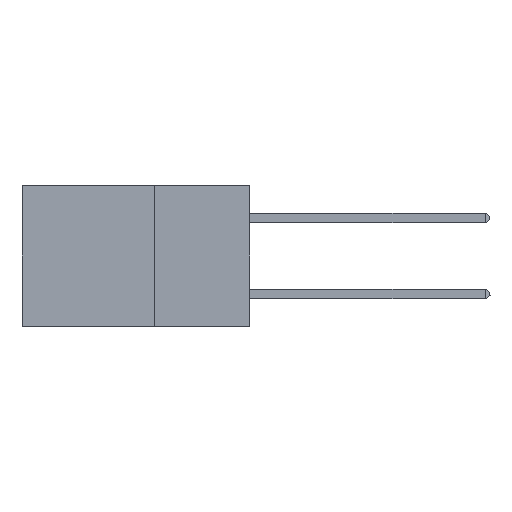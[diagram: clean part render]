
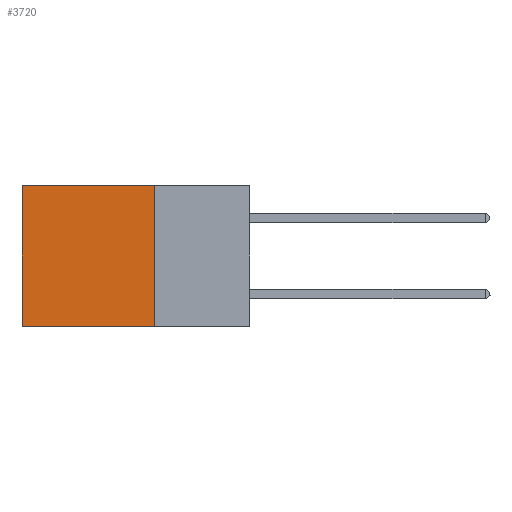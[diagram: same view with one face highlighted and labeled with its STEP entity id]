
A CAD part, left-side view. The second image highlights one B-rep face of the part: STEP entity #3720.
In plain terms, the highlighted planar face has unit normal (-1, 0, 0).
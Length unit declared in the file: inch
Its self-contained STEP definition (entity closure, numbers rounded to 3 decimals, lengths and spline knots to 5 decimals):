
#134 = AXIS2_PLACEMENT_3D ( 'NONE', #7249, #31932, #17650 ) ;
#166 = DIRECTION ( 'NONE',  ( 0., 1., 0. ) ) ;
#2289 = LINE ( 'NONE', #3078, #29446 ) ;
#2624 = DIRECTION ( 'NONE',  ( 0., 0., -1. ) ) ;
#3078 = CARTESIAN_POINT ( 'NONE',  ( 0.2875, 0.6, 0. ) ) ;
#3720 = ADVANCED_FACE ( 'NONE', ( #19783 ), #28200, .F. ) ;
#4526 = LINE ( 'NONE', #14279, #24523 ) ;
#5958 = DIRECTION ( 'NONE',  ( 0., 0., -1. ) ) ;
#6497 = CARTESIAN_POINT ( 'NONE',  ( 0.2875, 0.25, -0.37 ) ) ;
#6656 = VERTEX_POINT ( 'NONE', #38641 ) ;
#6936 = LINE ( 'NONE', #45559, #13033 ) ;
#7249 = CARTESIAN_POINT ( 'NONE',  ( 0.2875, 0.25, 0. ) ) ;
#12676 = VERTEX_POINT ( 'NONE', #6497 ) ;
#13033 = VECTOR ( 'NONE', #32696, 39.37008 ) ;
#14279 = CARTESIAN_POINT ( 'NONE',  ( 0.2875, 0.25, -0.37 ) ) ;
#15276 = CARTESIAN_POINT ( 'NONE',  ( 0.2875, 0.6, -0.37 ) ) ;
#17650 = DIRECTION ( 'NONE',  ( 0., 0., -1. ) ) ;
#19783 = FACE_OUTER_BOUND ( 'NONE', #35398, .T. ) ;
#24523 = VECTOR ( 'NONE', #166, 39.37008 ) ;
#24844 = ORIENTED_EDGE ( 'NONE', *, *, #31701, .T. ) ;
#25284 = EDGE_CURVE ( 'NONE', #12676, #30657, #4526, .T. ) ;
#25399 = LINE ( 'NONE', #26927, #41994 ) ;
#26927 = CARTESIAN_POINT ( 'NONE',  ( 0.2875, 0.25, 0. ) ) ;
#27238 = EDGE_CURVE ( 'NONE', #33437, #12676, #25399, .T. ) ;
#28200 = PLANE ( 'NONE',  #134 ) ;
#29446 = VECTOR ( 'NONE', #2624, 39.37008 ) ;
#30657 = VERTEX_POINT ( 'NONE', #15276 ) ;
#31381 = CARTESIAN_POINT ( 'NONE',  ( 0.2875, 0.25, 0. ) ) ;
#31701 = EDGE_CURVE ( 'NONE', #33437, #6656, #6936, .T. ) ;
#31932 = DIRECTION ( 'NONE',  ( 1., 0., 0. ) ) ;
#32696 = DIRECTION ( 'NONE',  ( 0., 1., 0. ) ) ;
#33437 = VERTEX_POINT ( 'NONE', #31381 ) ;
#35398 = EDGE_LOOP ( 'NONE', ( #45263, #39953, #37555, #24844 ) ) ;
#37555 = ORIENTED_EDGE ( 'NONE', *, *, #27238, .F. ) ;
#38641 = CARTESIAN_POINT ( 'NONE',  ( 0.2875, 0.6, 0. ) ) ;
#39495 = EDGE_CURVE ( 'NONE', #6656, #30657, #2289, .T. ) ;
#39953 = ORIENTED_EDGE ( 'NONE', *, *, #25284, .F. ) ;
#41994 = VECTOR ( 'NONE', #5958, 39.37008 ) ;
#45263 = ORIENTED_EDGE ( 'NONE', *, *, #39495, .T. ) ;
#45559 = CARTESIAN_POINT ( 'NONE',  ( 0.2875, 0.25, 0. ) ) ;
